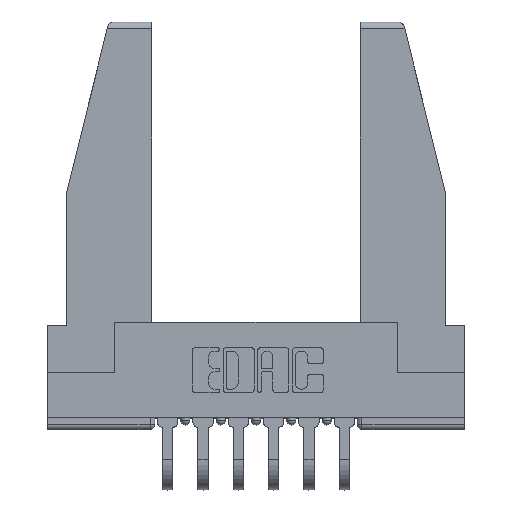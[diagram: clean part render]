
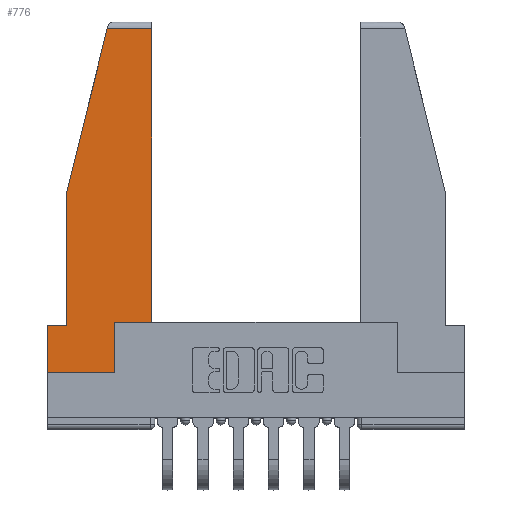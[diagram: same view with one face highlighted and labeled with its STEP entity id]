
A CAD part, top view. The second image highlights one B-rep face of the part: STEP entity #776.
In plain terms, the highlighted planar face has unit normal (0, 0, 1).
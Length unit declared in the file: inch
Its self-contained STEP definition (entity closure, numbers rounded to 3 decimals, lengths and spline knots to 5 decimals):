
#169 = DIRECTION ( 'NONE',  ( 0., 0., 1. ) ) ;
#260 = CARTESIAN_POINT ( 'NONE',  ( 0., 0.21, 0. ) ) ;
#266 = ORIENTED_EDGE ( 'NONE', *, *, #6186, .T. ) ;
#278 = LINE ( 'NONE', #10375, #9764 ) ;
#509 = DIRECTION ( 'NONE',  ( 1., 0., 0. ) ) ;
#776 = ADVANCED_FACE ( 'NONE', ( #11540 ), #4857, .T. ) ;
#998 = ORIENTED_EDGE ( 'NONE', *, *, #1875, .T. ) ;
#1123 = VERTEX_POINT ( 'NONE', #6711 ) ;
#1439 = LINE ( 'NONE', #6249, #7348 ) ;
#1514 = DIRECTION ( 'NONE',  ( -1., 0., 0. ) ) ;
#1813 = CARTESIAN_POINT ( 'NONE',  ( 0.297, 0., 0. ) ) ;
#1875 = EDGE_CURVE ( 'NONE', #7665, #11696, #3373, .T. ) ;
#2126 = LINE ( 'NONE', #5024, #11840 ) ;
#2496 = DIRECTION ( 'NONE',  ( 0., 1., 0. ) ) ;
#2618 = CARTESIAN_POINT ( 'NONE',  ( 0.086, 0.21, 0. ) ) ;
#3001 = LINE ( 'NONE', #5776, #6971 ) ;
#3039 = EDGE_CURVE ( 'NONE', #11138, #10035, #6383, .T. ) ;
#3071 = EDGE_CURVE ( 'NONE', #3141, #1123, #10128, .T. ) ;
#3141 = VERTEX_POINT ( 'NONE', #1813 ) ;
#3373 = LINE ( 'NONE', #7590, #8084 ) ;
#3620 = CARTESIAN_POINT ( 'NONE',  ( 0., 0.21, 0. ) ) ;
#3671 = LINE ( 'NONE', #6308, #8793 ) ;
#3928 = ORIENTED_EDGE ( 'NONE', *, *, #6859, .T. ) ;
#4116 = DIRECTION ( 'NONE',  ( -1., 0., 0. ) ) ;
#4313 = ORIENTED_EDGE ( 'NONE', *, *, #6248, .T. ) ;
#4857 = PLANE ( 'NONE',  #7869 ) ;
#5006 = EDGE_LOOP ( 'NONE', ( #11815, #266, #998, #9664, #6670, #3928, #4313, #11568, #10805 ) ) ;
#5024 = CARTESIAN_POINT ( 'NONE',  ( 0., 1.52, 0. ) ) ;
#5468 = VERTEX_POINT ( 'NONE', #9099 ) ;
#5776 = CARTESIAN_POINT ( 'NONE',  ( 0.086, 0.8, 0. ) ) ;
#6186 = EDGE_CURVE ( 'NONE', #8811, #7665, #2126, .T. ) ;
#6248 = EDGE_CURVE ( 'NONE', #6417, #3141, #1439, .T. ) ;
#6249 = CARTESIAN_POINT ( 'NONE',  ( 0., 0., 0. ) ) ;
#6308 = CARTESIAN_POINT ( 'NONE',  ( 0.461, 0.223, 0. ) ) ;
#6383 = LINE ( 'NONE', #3620, #7709 ) ;
#6417 = VERTEX_POINT ( 'NONE', #10236 ) ;
#6670 = ORIENTED_EDGE ( 'NONE', *, *, #3039, .T. ) ;
#6711 = CARTESIAN_POINT ( 'NONE',  ( 0.297, 0.223, 0. ) ) ;
#6859 = EDGE_CURVE ( 'NONE', #10035, #6417, #8553, .T. ) ;
#6931 = VECTOR ( 'NONE', #2496, 39.37008 ) ;
#6971 = VECTOR ( 'NONE', #9512, 39.37008 ) ;
#7348 = VECTOR ( 'NONE', #509, 39.37008 ) ;
#7385 = CARTESIAN_POINT ( 'NONE',  ( 0., 0.21, 0. ) ) ;
#7396 = EDGE_CURVE ( 'NONE', #11696, #11138, #3001, .T. ) ;
#7561 = CARTESIAN_POINT ( 'NONE',  ( 0., 0., 0. ) ) ;
#7590 = CARTESIAN_POINT ( 'NONE',  ( 0.271, 1.55, 0. ) ) ;
#7634 = DIRECTION ( 'NONE',  ( 0., -1., 0. ) ) ;
#7665 = VERTEX_POINT ( 'NONE', #10179 ) ;
#7709 = VECTOR ( 'NONE', #1514, 39.37008 ) ;
#7869 = AXIS2_PLACEMENT_3D ( 'NONE', #7561, #169, #11302 ) ;
#8084 = VECTOR ( 'NONE', #8574, 39.37008 ) ;
#8553 = LINE ( 'NONE', #7385, #11583 ) ;
#8574 = DIRECTION ( 'NONE',  ( -0.239, -0.971, 0. ) ) ;
#8599 = DIRECTION ( 'NONE',  ( 1., 0., 0. ) ) ;
#8793 = VECTOR ( 'NONE', #9312, 39.37008 ) ;
#8811 = VERTEX_POINT ( 'NONE', #9996 ) ;
#9099 = CARTESIAN_POINT ( 'NONE',  ( 0.461, 0.223, 0. ) ) ;
#9312 = DIRECTION ( 'NONE',  ( 0., 1., 0. ) ) ;
#9512 = DIRECTION ( 'NONE',  ( 0., -1., 0. ) ) ;
#9664 = ORIENTED_EDGE ( 'NONE', *, *, #7396, .T. ) ;
#9764 = VECTOR ( 'NONE', #8599, 39.37008 ) ;
#9996 = CARTESIAN_POINT ( 'NONE',  ( 0.461, 1.52, 0. ) ) ;
#10035 = VERTEX_POINT ( 'NONE', #260 ) ;
#10128 = LINE ( 'NONE', #11949, #6931 ) ;
#10179 = CARTESIAN_POINT ( 'NONE',  ( 0.2636, 1.52, 0. ) ) ;
#10236 = CARTESIAN_POINT ( 'NONE',  ( 0., 0., 0. ) ) ;
#10375 = CARTESIAN_POINT ( 'NONE',  ( 0.297, 0.223, 0. ) ) ;
#10805 = ORIENTED_EDGE ( 'NONE', *, *, #11316, .T. ) ;
#11138 = VERTEX_POINT ( 'NONE', #2618 ) ;
#11302 = DIRECTION ( 'NONE',  ( 1., 0., 0. ) ) ;
#11316 = EDGE_CURVE ( 'NONE', #1123, #5468, #278, .T. ) ;
#11540 = FACE_OUTER_BOUND ( 'NONE', #5006, .T. ) ;
#11568 = ORIENTED_EDGE ( 'NONE', *, *, #3071, .T. ) ;
#11583 = VECTOR ( 'NONE', #7634, 39.37008 ) ;
#11696 = VERTEX_POINT ( 'NONE', #12067 ) ;
#11707 = EDGE_CURVE ( 'NONE', #5468, #8811, #3671, .T. ) ;
#11815 = ORIENTED_EDGE ( 'NONE', *, *, #11707, .T. ) ;
#11840 = VECTOR ( 'NONE', #4116, 39.37008 ) ;
#11949 = CARTESIAN_POINT ( 'NONE',  ( 0.297, 0., 0. ) ) ;
#12067 = CARTESIAN_POINT ( 'NONE',  ( 0.086, 0.8, 0. ) ) ;
